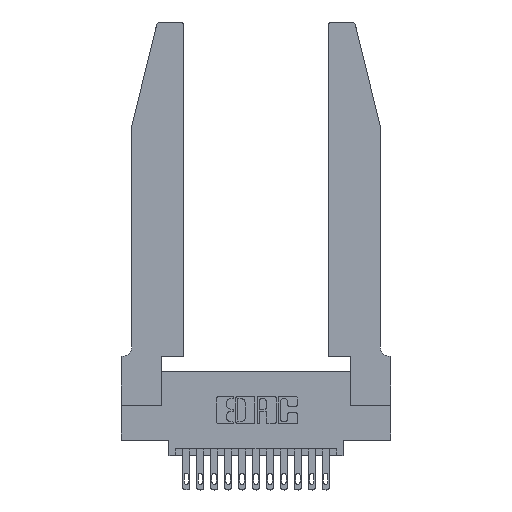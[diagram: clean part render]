
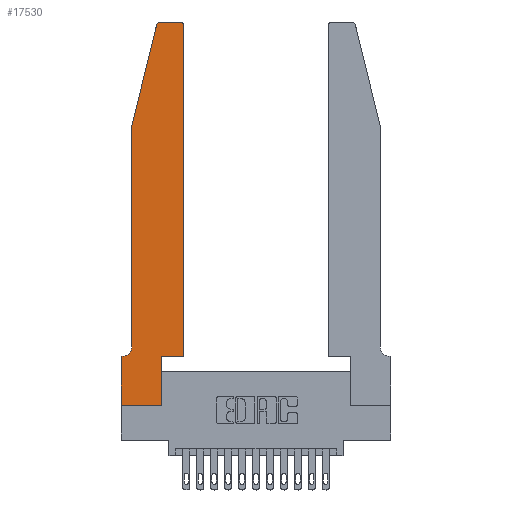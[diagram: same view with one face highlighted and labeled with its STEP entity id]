
A CAD part, top view. The second image highlights one B-rep face of the part: STEP entity #17530.
In plain terms, the highlighted planar face has unit normal (0, 0, 1).
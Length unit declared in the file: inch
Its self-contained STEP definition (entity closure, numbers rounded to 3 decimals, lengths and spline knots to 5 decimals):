
#573 = CARTESIAN_POINT ( 'NONE',  ( 0.2865, 0.35, 0.37 ) ) ;
#644 = EDGE_CURVE ( 'NONE', #16213, #15554, #2845, .T. ) ;
#971 = EDGE_CURVE ( 'NONE', #13840, #16895, #12130, .T. ) ;
#1290 = CARTESIAN_POINT ( 'NONE',  ( 0.4505, 0.35, 0.37 ) ) ;
#1348 = ORIENTED_EDGE ( 'NONE', *, *, #3229, .T. ) ;
#1509 = ORIENTED_EDGE ( 'NONE', *, *, #7421, .T. ) ;
#1526 = DIRECTION ( 'NONE',  ( 0., 1., 0. ) ) ;
#1853 = EDGE_CURVE ( 'NONE', #16895, #10186, #5605, .T. ) ;
#2108 = CARTESIAN_POINT ( 'NONE',  ( 0., 0., 0.37 ) ) ;
#2237 = DIRECTION ( 'NONE',  ( 1., 0., 0. ) ) ;
#2579 = LINE ( 'NONE', #12673, #4502 ) ;
#2641 = CIRCLE ( 'NONE', #12250, 0.03 ) ;
#2845 = LINE ( 'NONE', #1290, #6881 ) ;
#3195 = PLANE ( 'NONE',  #13809 ) ;
#3229 = EDGE_CURVE ( 'NONE', #10604, #6448, #12082, .T. ) ;
#3347 = DIRECTION ( 'NONE',  ( 0., -1., 0. ) ) ;
#3428 = VERTEX_POINT ( 'NONE', #10980 ) ;
#3439 = CARTESIAN_POINT ( 'NONE',  ( 0.4205, 2.72, 0.37 ) ) ;
#3941 = CARTESIAN_POINT ( 'NONE',  ( 0.4505, 0.35, 0.37 ) ) ;
#4050 = CARTESIAN_POINT ( 'NONE',  ( 0.284, 2.72, 0.37 ) ) ;
#4227 = VECTOR ( 'NONE', #1526, 39.37008 ) ;
#4278 = VECTOR ( 'NONE', #11158, 39.37008 ) ;
#4334 = VECTOR ( 'NONE', #3347, 39.37008 ) ;
#4401 = CARTESIAN_POINT ( 'NONE',  ( 0.2605, 2.75, 0.37 ) ) ;
#4502 = VECTOR ( 'NONE', #13814, 39.37008 ) ;
#5255 = EDGE_CURVE ( 'NONE', #5426, #5460, #17179, .T. ) ;
#5426 = VERTEX_POINT ( 'NONE', #6464 ) ;
#5460 = VERTEX_POINT ( 'NONE', #17225 ) ;
#5501 = CARTESIAN_POINT ( 'NONE',  ( 0.0755, 2., 0.37 ) ) ;
#5605 = CIRCLE ( 'NONE', #10197, 0.07 ) ;
#5957 = DIRECTION ( 'NONE',  ( -1., 0., 0. ) ) ;
#6230 = VERTEX_POINT ( 'NONE', #7060 ) ;
#6264 = DIRECTION ( 'NONE',  ( 0., -1., 0. ) ) ;
#6448 = VERTEX_POINT ( 'NONE', #15520 ) ;
#6464 = CARTESIAN_POINT ( 'NONE',  ( 0.284, 2.75, 0.37 ) ) ;
#6881 = VECTOR ( 'NONE', #8062, 39.37008 ) ;
#7060 = CARTESIAN_POINT ( 'NONE',  ( 0., 0.35, 0.37 ) ) ;
#7123 = DIRECTION ( 'NONE',  ( 1., 0., 0. ) ) ;
#7219 = LINE ( 'NONE', #9838, #4278 ) ;
#7296 = LINE ( 'NONE', #2108, #4334 ) ;
#7374 = FACE_OUTER_BOUND ( 'NONE', #7376, .T. ) ;
#7376 = EDGE_LOOP ( 'NONE', ( #15792, #16494, #1509, #13487, #13953, #9975, #15468, #1348, #10953, #7631, #9780, #12992 ) ) ;
#7421 = EDGE_CURVE ( 'NONE', #5460, #13840, #7219, .T. ) ;
#7551 = EDGE_CURVE ( 'NONE', #6448, #16213, #15307, .T. ) ;
#7631 = ORIENTED_EDGE ( 'NONE', *, *, #644, .T. ) ;
#8062 = DIRECTION ( 'NONE',  ( 1., 0., 0. ) ) ;
#8445 = DIRECTION ( 'NONE',  ( 0., 0., 1. ) ) ;
#8589 = VECTOR ( 'NONE', #6264, 39.37008 ) ;
#8925 = DIRECTION ( 'NONE',  ( 0., 0., 1. ) ) ;
#9257 = CARTESIAN_POINT ( 'NONE',  ( 0.0055, 0.35, 0.37 ) ) ;
#9780 = ORIENTED_EDGE ( 'NONE', *, *, #13847, .T. ) ;
#9838 = CARTESIAN_POINT ( 'NONE',  ( 0.0755, 2., 0.37 ) ) ;
#9975 = ORIENTED_EDGE ( 'NONE', *, *, #15161, .T. ) ;
#10186 = VERTEX_POINT ( 'NONE', #9257 ) ;
#10197 = AXIS2_PLACEMENT_3D ( 'NONE', #13455, #12548, #5957 ) ;
#10389 = EDGE_CURVE ( 'NONE', #3428, #5426, #12823, .T. ) ;
#10415 = VERTEX_POINT ( 'NONE', #12500 ) ;
#10542 = LINE ( 'NONE', #13590, #4227 ) ;
#10604 = VERTEX_POINT ( 'NONE', #15820 ) ;
#10953 = ORIENTED_EDGE ( 'NONE', *, *, #7551, .T. ) ;
#10980 = CARTESIAN_POINT ( 'NONE',  ( 0.4205, 2.75, 0.37 ) ) ;
#11158 = DIRECTION ( 'NONE',  ( -0.239, -0.971, 0. ) ) ;
#11277 = DIRECTION ( 'NONE',  ( 1., 0., 0. ) ) ;
#11634 = VECTOR ( 'NONE', #15663, 39.37008 ) ;
#11691 = CARTESIAN_POINT ( 'NONE',  ( 0., 0., 0.37 ) ) ;
#11777 = EDGE_CURVE ( 'NONE', #10415, #3428, #2641, .T. ) ;
#12082 = LINE ( 'NONE', #11691, #16815 ) ;
#12130 = LINE ( 'NONE', #17080, #8589 ) ;
#12250 = AXIS2_PLACEMENT_3D ( 'NONE', #3439, #8925, #13354 ) ;
#12500 = CARTESIAN_POINT ( 'NONE',  ( 0.4505, 2.72, 0.37 ) ) ;
#12548 = DIRECTION ( 'NONE',  ( 0., 0., -1. ) ) ;
#12654 = CARTESIAN_POINT ( 'NONE',  ( 0., 0.35, 0.37 ) ) ;
#12673 = CARTESIAN_POINT ( 'NONE',  ( 0.0755, 0.35, 0.37 ) ) ;
#12823 = LINE ( 'NONE', #4401, #14560 ) ;
#12992 = ORIENTED_EDGE ( 'NONE', *, *, #11777, .T. ) ;
#13354 = DIRECTION ( 'NONE',  ( 1., 0., 0. ) ) ;
#13455 = CARTESIAN_POINT ( 'NONE',  ( 0.0055, 0.42, 0.37 ) ) ;
#13487 = ORIENTED_EDGE ( 'NONE', *, *, #971, .T. ) ;
#13590 = CARTESIAN_POINT ( 'NONE',  ( 0.4505, 0.35, 0.37 ) ) ;
#13809 = AXIS2_PLACEMENT_3D ( 'NONE', #12654, #8445, #7123 ) ;
#13814 = DIRECTION ( 'NONE',  ( -1., 0., 0. ) ) ;
#13840 = VERTEX_POINT ( 'NONE', #5501 ) ;
#13847 = EDGE_CURVE ( 'NONE', #15554, #10415, #10542, .T. ) ;
#13953 = ORIENTED_EDGE ( 'NONE', *, *, #1853, .T. ) ;
#14045 = EDGE_CURVE ( 'NONE', #6230, #10604, #7296, .T. ) ;
#14560 = VECTOR ( 'NONE', #16365, 39.37008 ) ;
#14761 = DIRECTION ( 'NONE',  ( 0., 0., 1. ) ) ;
#15161 = EDGE_CURVE ( 'NONE', #10186, #6230, #2579, .T. ) ;
#15292 = CARTESIAN_POINT ( 'NONE',  ( 0.0755, 0.42, 0.37 ) ) ;
#15307 = LINE ( 'NONE', #573, #11634 ) ;
#15468 = ORIENTED_EDGE ( 'NONE', *, *, #14045, .T. ) ;
#15520 = CARTESIAN_POINT ( 'NONE',  ( 0.2865, 0., 0.37 ) ) ;
#15550 = AXIS2_PLACEMENT_3D ( 'NONE', #4050, #14761, #11277 ) ;
#15554 = VERTEX_POINT ( 'NONE', #3941 ) ;
#15663 = DIRECTION ( 'NONE',  ( 0., 1., 0. ) ) ;
#15792 = ORIENTED_EDGE ( 'NONE', *, *, #10389, .T. ) ;
#15820 = CARTESIAN_POINT ( 'NONE',  ( 0., 0., 0.37 ) ) ;
#16198 = CARTESIAN_POINT ( 'NONE',  ( 0.2865, 0.35, 0.37 ) ) ;
#16213 = VERTEX_POINT ( 'NONE', #16198 ) ;
#16365 = DIRECTION ( 'NONE',  ( -1., 0., 0. ) ) ;
#16494 = ORIENTED_EDGE ( 'NONE', *, *, #5255, .T. ) ;
#16815 = VECTOR ( 'NONE', #2237, 39.37008 ) ;
#16895 = VERTEX_POINT ( 'NONE', #15292 ) ;
#17080 = CARTESIAN_POINT ( 'NONE',  ( 0.0755, 2., 0.37 ) ) ;
#17179 = CIRCLE ( 'NONE', #15550, 0.03 ) ;
#17225 = CARTESIAN_POINT ( 'NONE',  ( 0.25487, 2.72718, 0.37 ) ) ;
#17530 = ADVANCED_FACE ( 'NONE', ( #7374 ), #3195, .T. ) ;
